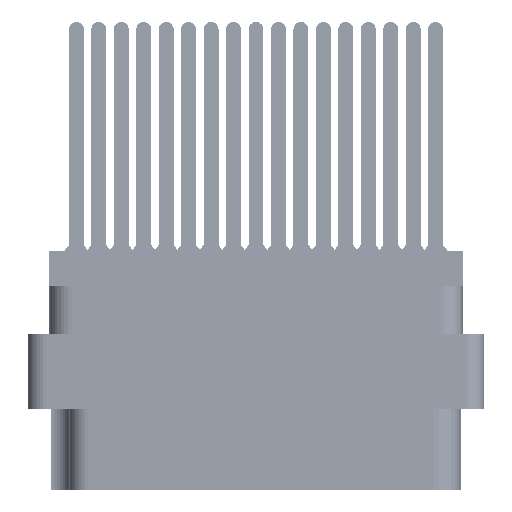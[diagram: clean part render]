
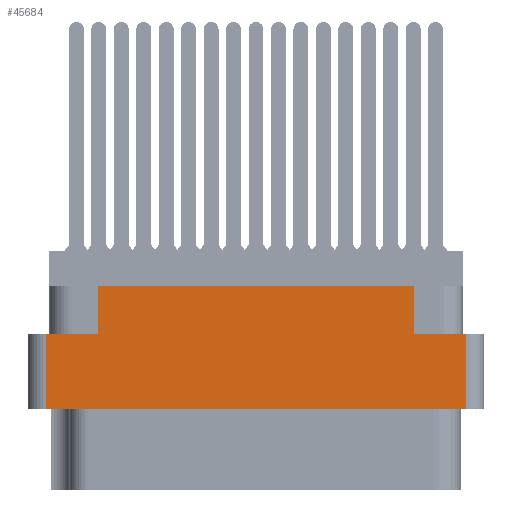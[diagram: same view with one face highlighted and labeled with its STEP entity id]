
A CAD part, left-side view. The second image highlights one B-rep face of the part: STEP entity #45684.
In plain terms, the highlighted planar face has unit normal (-1, 0, 0).
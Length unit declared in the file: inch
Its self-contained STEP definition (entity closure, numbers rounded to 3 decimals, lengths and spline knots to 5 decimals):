
#5546 = DIRECTION ( 'NONE',  ( 0., 0., 1. ) ) ;
#6302 = LINE ( 'NONE', #49960, #79054 ) ;
#6372 = EDGE_CURVE ( 'NONE', #17384, #14936, #54479, .T. ) ;
#6511 = EDGE_CURVE ( 'NONE', #45196, #9801, #36339, .T. ) ;
#6590 = LINE ( 'NONE', #62712, #54346 ) ;
#7125 = DIRECTION ( 'NONE',  ( 0., -1., 0. ) ) ;
#8903 = VERTEX_POINT ( 'NONE', #64185 ) ;
#9801 = VERTEX_POINT ( 'NONE', #62889 ) ;
#9819 = CARTESIAN_POINT ( 'NONE',  ( -1.375, 0.7005, -0.798 ) ) ;
#10282 = EDGE_CURVE ( 'NONE', #17384, #32579, #16143, .T. ) ;
#10701 = CARTESIAN_POINT ( 'NONE',  ( -1.375, 0.5285, -0.277 ) ) ;
#12548 = VECTOR ( 'NONE', #71605, 39.37008 ) ;
#13299 = FACE_OUTER_BOUND ( 'NONE', #26061, .T. ) ;
#14785 = CARTESIAN_POINT ( 'NONE',  ( -1.375, 0., -0.277 ) ) ;
#14936 = VERTEX_POINT ( 'NONE', #73738 ) ;
#16143 = LINE ( 'NONE', #25984, #25264 ) ;
#17384 = VERTEX_POINT ( 'NONE', #92155 ) ;
#21656 = EDGE_CURVE ( 'NONE', #32579, #45196, #61366, .T. ) ;
#22682 = VERTEX_POINT ( 'NONE', #83126 ) ;
#22906 = LINE ( 'NONE', #33342, #54672 ) ;
#25264 = VECTOR ( 'NONE', #47595, 39.37008 ) ;
#25572 = ORIENTED_EDGE ( 'NONE', *, *, #80955, .F. ) ;
#25984 = CARTESIAN_POINT ( 'NONE',  ( -1.375, 0., -0.277 ) ) ;
#26061 = EDGE_LOOP ( 'NONE', ( #79822, #30469, #25572, #90592, #83723, #30348, #52302, #65866 ) ) ;
#26632 = DIRECTION ( 'NONE',  ( 0., 0., 1. ) ) ;
#28988 = DIRECTION ( 'NONE',  ( 0., 1., 0. ) ) ;
#29126 = EDGE_CURVE ( 'NONE', #39186, #8903, #6590, .T. ) ;
#30345 = EDGE_CURVE ( 'NONE', #22682, #9801, #22906, .T. ) ;
#30348 = ORIENTED_EDGE ( 'NONE', *, *, #30345, .T. ) ;
#30469 = ORIENTED_EDGE ( 'NONE', *, *, #6372, .T. ) ;
#31197 = EDGE_CURVE ( 'NONE', #22682, #8903, #82850, .T. ) ;
#32579 = VERTEX_POINT ( 'NONE', #10701 ) ;
#33342 = CARTESIAN_POINT ( 'NONE',  ( -1.375, -0.5285, -0.277 ) ) ;
#34025 = VECTOR ( 'NONE', #53953, 39.37008 ) ;
#36339 = LINE ( 'NONE', #48889, #51054 ) ;
#39186 = VERTEX_POINT ( 'NONE', #45233 ) ;
#40600 = CARTESIAN_POINT ( 'NONE',  ( -1.375, -0.7625, -0.798 ) ) ;
#40877 = DIRECTION ( 'NONE',  ( 0., 0., 1. ) ) ;
#41868 = DIRECTION ( 'NONE',  ( -1., 0., 0. ) ) ;
#45196 = VERTEX_POINT ( 'NONE', #73252 ) ;
#45233 = CARTESIAN_POINT ( 'NONE',  ( -1.375, -0.7005, -0.529 ) ) ;
#45684 = ADVANCED_FACE ( 'NONE', ( #13299 ), #63063, .T. ) ;
#47595 = DIRECTION ( 'NONE',  ( 0., -1., 0. ) ) ;
#47731 = AXIS2_PLACEMENT_3D ( 'NONE', #40600, #41868, #5546 ) ;
#48889 = CARTESIAN_POINT ( 'NONE',  ( -1.375, 0.7625, -0.117 ) ) ;
#49960 = CARTESIAN_POINT ( 'NONE',  ( -1.375, 0., -0.529 ) ) ;
#51054 = VECTOR ( 'NONE', #63766, 39.37008 ) ;
#52302 = ORIENTED_EDGE ( 'NONE', *, *, #6511, .F. ) ;
#53953 = DIRECTION ( 'NONE',  ( 0., 0., -1. ) ) ;
#54346 = VECTOR ( 'NONE', #40877, 39.37008 ) ;
#54479 = LINE ( 'NONE', #9819, #34025 ) ;
#54672 = VECTOR ( 'NONE', #26632, 39.37008 ) ;
#61366 = LINE ( 'NONE', #78600, #12548 ) ;
#62712 = CARTESIAN_POINT ( 'NONE',  ( -1.375, -0.7005, -0.798 ) ) ;
#62889 = CARTESIAN_POINT ( 'NONE',  ( -1.375, -0.5285, -0.117 ) ) ;
#63063 = PLANE ( 'NONE',  #47731 ) ;
#63766 = DIRECTION ( 'NONE',  ( 0., -1., 0. ) ) ;
#64185 = CARTESIAN_POINT ( 'NONE',  ( -1.375, -0.7005, -0.277 ) ) ;
#65866 = ORIENTED_EDGE ( 'NONE', *, *, #21656, .F. ) ;
#70315 = VECTOR ( 'NONE', #7125, 39.37008 ) ;
#71605 = DIRECTION ( 'NONE',  ( 0., 0., 1. ) ) ;
#73252 = CARTESIAN_POINT ( 'NONE',  ( -1.375, 0.5285, -0.117 ) ) ;
#73738 = CARTESIAN_POINT ( 'NONE',  ( -1.375, 0.7005, -0.529 ) ) ;
#78600 = CARTESIAN_POINT ( 'NONE',  ( -1.375, 0.5285, -0.277 ) ) ;
#79054 = VECTOR ( 'NONE', #28988, 39.37008 ) ;
#79822 = ORIENTED_EDGE ( 'NONE', *, *, #10282, .F. ) ;
#80955 = EDGE_CURVE ( 'NONE', #39186, #14936, #6302, .T. ) ;
#82850 = LINE ( 'NONE', #14785, #70315 ) ;
#83126 = CARTESIAN_POINT ( 'NONE',  ( -1.375, -0.5285, -0.277 ) ) ;
#83723 = ORIENTED_EDGE ( 'NONE', *, *, #31197, .F. ) ;
#90592 = ORIENTED_EDGE ( 'NONE', *, *, #29126, .T. ) ;
#92155 = CARTESIAN_POINT ( 'NONE',  ( -1.375, 0.7005, -0.277 ) ) ;
